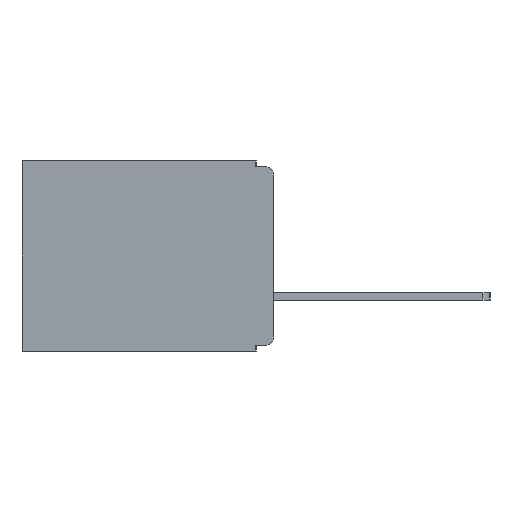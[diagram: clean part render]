
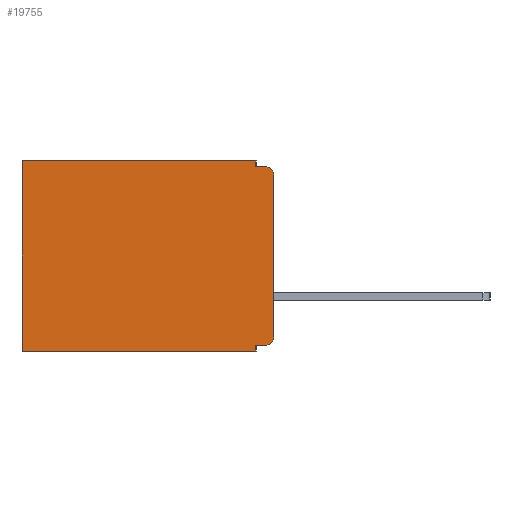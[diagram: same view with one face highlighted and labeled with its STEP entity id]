
A CAD part, left-side view. The second image highlights one B-rep face of the part: STEP entity #19755.
In plain terms, the highlighted planar face has unit normal (-1, 0, 0).
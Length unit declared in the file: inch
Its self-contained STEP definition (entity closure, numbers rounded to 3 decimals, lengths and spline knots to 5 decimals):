
#449 = CARTESIAN_POINT ( 'NONE',  ( 0.3, 0., -0.01 ) ) ;
#501 = VERTEX_POINT ( 'NONE', #18028 ) ;
#502 = CIRCLE ( 'NONE', #19810, 0.015 ) ;
#773 = VERTEX_POINT ( 'NONE', #16965 ) ;
#1023 = DIRECTION ( 'NONE',  ( 0., 0., -1. ) ) ;
#1164 = DIRECTION ( 'NONE',  ( 0., 1., 0. ) ) ;
#1361 = LINE ( 'NONE', #9328, #10705 ) ;
#2032 = CARTESIAN_POINT ( 'NONE',  ( 0.3, 0.031, -0.01 ) ) ;
#2049 = FACE_OUTER_BOUND ( 'NONE', #23838, .T. ) ;
#2167 = DIRECTION ( 'NONE',  ( 0., 0., -1. ) ) ;
#2242 = VECTOR ( 'NONE', #1023, 39.37008 ) ;
#2271 = VERTEX_POINT ( 'NONE', #12598 ) ;
#2298 = DIRECTION ( 'NONE',  ( 0., -1., 0. ) ) ;
#2497 = CARTESIAN_POINT ( 'NONE',  ( 0.3, 0.015, -0.01 ) ) ;
#2701 = CARTESIAN_POINT ( 'NONE',  ( 0.3, 0., -0.025 ) ) ;
#3170 = EDGE_CURVE ( 'NONE', #5864, #17276, #14841, .T. ) ;
#3202 = VECTOR ( 'NONE', #1164, 39.37008 ) ;
#3204 = DIRECTION ( 'NONE',  ( 1., 0., 0. ) ) ;
#3404 = ORIENTED_EDGE ( 'NONE', *, *, #14196, .T. ) ;
#4088 = EDGE_CURVE ( 'NONE', #18914, #18905, #14213, .T. ) ;
#4874 = DIRECTION ( 'NONE',  ( 0., 0., -1. ) ) ;
#5061 = CARTESIAN_POINT ( 'NONE',  ( 0.3, 0.031, 0. ) ) ;
#5421 = ORIENTED_EDGE ( 'NONE', *, *, #7779, .F. ) ;
#5718 = EDGE_CURVE ( 'NONE', #9750, #8132, #12080, .T. ) ;
#5864 = VERTEX_POINT ( 'NONE', #2701 ) ;
#5946 = VECTOR ( 'NONE', #2298, 39.37008 ) ;
#6204 = CARTESIAN_POINT ( 'NONE',  ( 0.3, 0.031, -0.32 ) ) ;
#6540 = CARTESIAN_POINT ( 'NONE',  ( 0.3, 0.031, 0. ) ) ;
#6686 = CARTESIAN_POINT ( 'NONE',  ( 0.3, 0.015, -0.025 ) ) ;
#7197 = VERTEX_POINT ( 'NONE', #5061 ) ;
#7368 = AXIS2_PLACEMENT_3D ( 'NONE', #14385, #3204, #16272 ) ;
#7534 = ORIENTED_EDGE ( 'NONE', *, *, #22444, .T. ) ;
#7779 = EDGE_CURVE ( 'NONE', #18905, #501, #18087, .T. ) ;
#7800 = LINE ( 'NONE', #6540, #2242 ) ;
#8132 = VERTEX_POINT ( 'NONE', #2497 ) ;
#8591 = DIRECTION ( 'NONE',  ( 0., 0., -1. ) ) ;
#8643 = CARTESIAN_POINT ( 'NONE',  ( 0.3, 0., -0.33 ) ) ;
#8804 = DIRECTION ( 'NONE',  ( 0., 1., 0. ) ) ;
#9328 = CARTESIAN_POINT ( 'NONE',  ( 0.3, 0., -0.32 ) ) ;
#9564 = ORIENTED_EDGE ( 'NONE', *, *, #11915, .F. ) ;
#9750 = VERTEX_POINT ( 'NONE', #2032 ) ;
#10144 = CARTESIAN_POINT ( 'NONE',  ( 0.3, 0.015, -0.305 ) ) ;
#10491 = VECTOR ( 'NONE', #4874, 39.37008 ) ;
#10664 = PLANE ( 'NONE',  #7368 ) ;
#10705 = VECTOR ( 'NONE', #11200, 39.37008 ) ;
#10785 = LINE ( 'NONE', #21839, #16308 ) ;
#11075 = AXIS2_PLACEMENT_3D ( 'NONE', #10144, #23165, #12010 ) ;
#11200 = DIRECTION ( 'NONE',  ( 0., 1., 0. ) ) ;
#11356 = CARTESIAN_POINT ( 'NONE',  ( 0.3, 0.437, -0.33 ) ) ;
#11423 = ORIENTED_EDGE ( 'NONE', *, *, #3170, .F. ) ;
#11633 = EDGE_CURVE ( 'NONE', #7197, #9750, #7800, .T. ) ;
#11915 = EDGE_CURVE ( 'NONE', #2271, #18914, #1361, .T. ) ;
#12010 = DIRECTION ( 'NONE',  ( 0., 0., -1. ) ) ;
#12080 = LINE ( 'NONE', #449, #5946 ) ;
#12148 = CIRCLE ( 'NONE', #11075, 0.015 ) ;
#12598 = CARTESIAN_POINT ( 'NONE',  ( 0.3, 0.015, -0.32 ) ) ;
#13018 = ORIENTED_EDGE ( 'NONE', *, *, #4088, .F. ) ;
#13650 = CARTESIAN_POINT ( 'NONE',  ( 0.3, 0.031, -0.33 ) ) ;
#14033 = CARTESIAN_POINT ( 'NONE',  ( 0.3, 0., -0.305 ) ) ;
#14196 = EDGE_CURVE ( 'NONE', #7197, #773, #10785, .T. ) ;
#14213 = LINE ( 'NONE', #22611, #19156 ) ;
#14385 = CARTESIAN_POINT ( 'NONE',  ( 0.3, 0., -0.33 ) ) ;
#14841 = LINE ( 'NONE', #8643, #10491 ) ;
#16272 = DIRECTION ( 'NONE',  ( 0., 0., -1. ) ) ;
#16308 = VECTOR ( 'NONE', #8804, 39.37008 ) ;
#16507 = VECTOR ( 'NONE', #22510, 39.37008 ) ;
#16965 = CARTESIAN_POINT ( 'NONE',  ( 0.3, 0.437, 0. ) ) ;
#17276 = VERTEX_POINT ( 'NONE', #14033 ) ;
#18028 = CARTESIAN_POINT ( 'NONE',  ( 0.3, 0.437, -0.33 ) ) ;
#18087 = LINE ( 'NONE', #21615, #3202 ) ;
#18600 = ORIENTED_EDGE ( 'NONE', *, *, #22883, .T. ) ;
#18905 = VERTEX_POINT ( 'NONE', #13650 ) ;
#18914 = VERTEX_POINT ( 'NONE', #6204 ) ;
#19156 = VECTOR ( 'NONE', #2167, 39.37008 ) ;
#19742 = DIRECTION ( 'NONE',  ( -1., 0., 0. ) ) ;
#19755 = ADVANCED_FACE ( 'NONE', ( #2049 ), #10664, .F. ) ;
#19801 = ORIENTED_EDGE ( 'NONE', *, *, #22545, .T. ) ;
#19810 = AXIS2_PLACEMENT_3D ( 'NONE', #6686, #19742, #8591 ) ;
#21467 = LINE ( 'NONE', #11356, #16507 ) ;
#21615 = CARTESIAN_POINT ( 'NONE',  ( 0.3, 0., -0.33 ) ) ;
#21839 = CARTESIAN_POINT ( 'NONE',  ( 0.3, 0., 0. ) ) ;
#22444 = EDGE_CURVE ( 'NONE', #2271, #17276, #12148, .T. ) ;
#22453 = ORIENTED_EDGE ( 'NONE', *, *, #5718, .F. ) ;
#22510 = DIRECTION ( 'NONE',  ( 0., 0., -1. ) ) ;
#22545 = EDGE_CURVE ( 'NONE', #5864, #8132, #502, .T. ) ;
#22611 = CARTESIAN_POINT ( 'NONE',  ( 0.3, 0.031, -0.33 ) ) ;
#22883 = EDGE_CURVE ( 'NONE', #773, #501, #21467, .T. ) ;
#23165 = DIRECTION ( 'NONE',  ( -1., 0., 0. ) ) ;
#23838 = EDGE_LOOP ( 'NONE', ( #11423, #19801, #22453, #24103, #3404, #18600, #5421, #13018, #9564, #7534 ) ) ;
#24103 = ORIENTED_EDGE ( 'NONE', *, *, #11633, .F. ) ;
